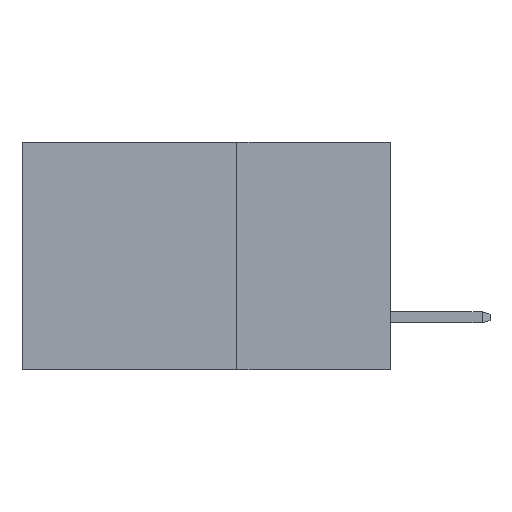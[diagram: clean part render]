
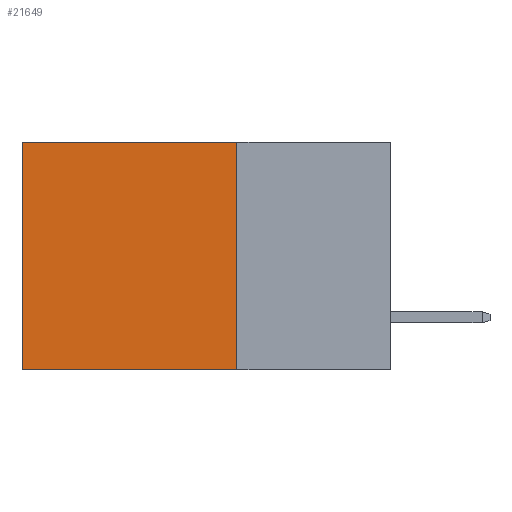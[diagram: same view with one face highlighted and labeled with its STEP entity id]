
A CAD part, left-side view. The second image highlights one B-rep face of the part: STEP entity #21649.
In plain terms, the highlighted planar face has unit normal (-1, 0, 0).
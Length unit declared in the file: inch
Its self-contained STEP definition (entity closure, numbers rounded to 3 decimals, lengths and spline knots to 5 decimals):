
#183 = DIRECTION ( 'NONE',  ( 0., 1., 0. ) ) ;
#2206 = VECTOR ( 'NONE', #183, 39.37008 ) ;
#4807 = EDGE_CURVE ( 'NONE', #10448, #7651, #21077, .T. ) ;
#5184 = EDGE_CURVE ( 'NONE', #16431, #10448, #13980, .T. ) ;
#5535 = CARTESIAN_POINT ( 'NONE',  ( 0.2875, 0.25, 0. ) ) ;
#5704 = CARTESIAN_POINT ( 'NONE',  ( 0.2875, 0.25, 0. ) ) ;
#6079 = CARTESIAN_POINT ( 'NONE',  ( 0.2875, 0.25, 0. ) ) ;
#6943 = VECTOR ( 'NONE', #11288, 39.37008 ) ;
#6973 = CARTESIAN_POINT ( 'NONE',  ( 0.2875, 0.25, -0.37 ) ) ;
#7651 = VERTEX_POINT ( 'NONE', #10925 ) ;
#7995 = LINE ( 'NONE', #6079, #6943 ) ;
#8091 = ORIENTED_EDGE ( 'NONE', *, *, #20629, .F. ) ;
#8295 = EDGE_CURVE ( 'NONE', #16700, #7651, #16976, .T. ) ;
#8610 = DIRECTION ( 'NONE',  ( 0., 0., -1. ) ) ;
#8966 = CARTESIAN_POINT ( 'NONE',  ( 0.2875, 0.6, 0. ) ) ;
#9574 = DIRECTION ( 'NONE',  ( 0., 1., 0. ) ) ;
#10230 = DIRECTION ( 'NONE',  ( 1., 0., 0. ) ) ;
#10448 = VERTEX_POINT ( 'NONE', #8966 ) ;
#10711 = ORIENTED_EDGE ( 'NONE', *, *, #5184, .T. ) ;
#10925 = CARTESIAN_POINT ( 'NONE',  ( 0.2875, 0.6, -0.37 ) ) ;
#11288 = DIRECTION ( 'NONE',  ( 0., 0., -1. ) ) ;
#11351 = ORIENTED_EDGE ( 'NONE', *, *, #8295, .F. ) ;
#11568 = ORIENTED_EDGE ( 'NONE', *, *, #4807, .T. ) ;
#13980 = LINE ( 'NONE', #16852, #2206 ) ;
#14000 = EDGE_LOOP ( 'NONE', ( #11568, #11351, #8091, #10711 ) ) ;
#15398 = DIRECTION ( 'NONE',  ( 0., 0., -1. ) ) ;
#16431 = VERTEX_POINT ( 'NONE', #5704 ) ;
#16700 = VERTEX_POINT ( 'NONE', #6973 ) ;
#16852 = CARTESIAN_POINT ( 'NONE',  ( 0.2875, 0.25, 0. ) ) ;
#16976 = LINE ( 'NONE', #17915, #19113 ) ;
#17915 = CARTESIAN_POINT ( 'NONE',  ( 0.2875, 0.25, -0.37 ) ) ;
#18145 = VECTOR ( 'NONE', #15398, 39.37008 ) ;
#18808 = PLANE ( 'NONE',  #21740 ) ;
#19113 = VECTOR ( 'NONE', #9574, 39.37008 ) ;
#20226 = CARTESIAN_POINT ( 'NONE',  ( 0.2875, 0.6, 0. ) ) ;
#20583 = FACE_OUTER_BOUND ( 'NONE', #14000, .T. ) ;
#20629 = EDGE_CURVE ( 'NONE', #16431, #16700, #7995, .T. ) ;
#21077 = LINE ( 'NONE', #20226, #18145 ) ;
#21649 = ADVANCED_FACE ( 'NONE', ( #20583 ), #18808, .F. ) ;
#21740 = AXIS2_PLACEMENT_3D ( 'NONE', #5535, #10230, #8610 ) ;
